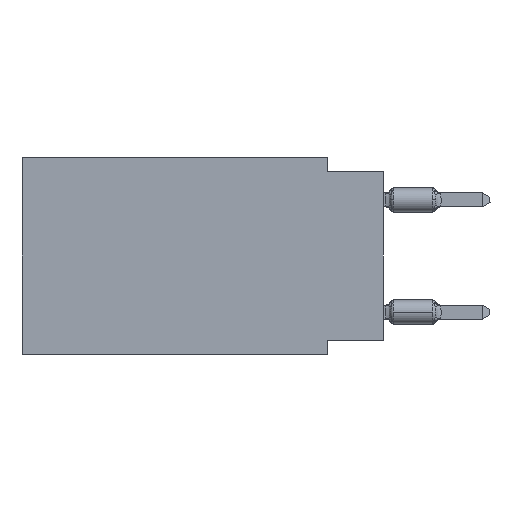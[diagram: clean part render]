
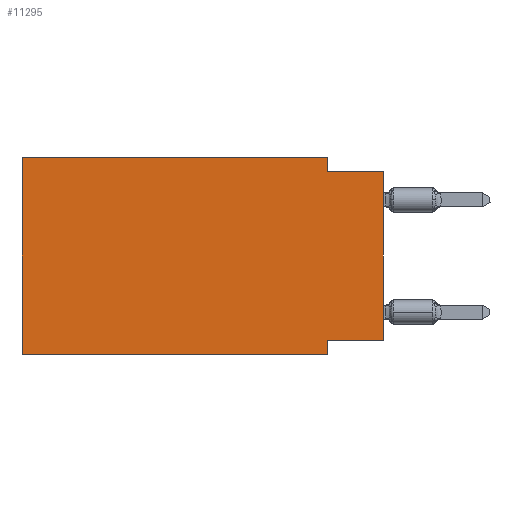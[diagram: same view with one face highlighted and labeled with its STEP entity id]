
A CAD part, left-side view. The second image highlights one B-rep face of the part: STEP entity #11295.
In plain terms, the highlighted planar face has unit normal (-1, 0, 0).
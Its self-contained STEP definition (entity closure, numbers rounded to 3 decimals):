
#116 = LINE ( 'NONE', #10203, #14946 ) ;
#575 = CARTESIAN_POINT ( 'NONE',  ( 0., 16.383, 0. ) ) ;
#640 = CARTESIAN_POINT ( 'NONE',  ( 0., 0., -0.635 ) ) ;
#756 = CARTESIAN_POINT ( 'NONE',  ( 0., 16.383, 0. ) ) ;
#851 = VERTEX_POINT ( 'NONE', #13992 ) ;
#1028 = CARTESIAN_POINT ( 'NONE',  ( 0., 16.383, -8.89 ) ) ;
#1067 = DIRECTION ( 'NONE',  ( 0., 0., -1. ) ) ;
#1612 = ORIENTED_EDGE ( 'NONE', *, *, #9299, .T. ) ;
#1978 = CARTESIAN_POINT ( 'NONE',  ( 0., 0., -8.255 ) ) ;
#2279 = LINE ( 'NONE', #756, #11150 ) ;
#2383 = CARTESIAN_POINT ( 'NONE',  ( 0., 2.54, -8.89 ) ) ;
#2722 = CARTESIAN_POINT ( 'NONE',  ( 0., 16.383, 0. ) ) ;
#2803 = VECTOR ( 'NONE', #16904, 1000. ) ;
#2999 = LINE ( 'NONE', #9617, #2803 ) ;
#3712 = CARTESIAN_POINT ( 'NONE',  ( 0., 16.383, -8.89 ) ) ;
#4449 = VERTEX_POINT ( 'NONE', #640 ) ;
#5041 = CARTESIAN_POINT ( 'NONE',  ( 0., 16.383, 0. ) ) ;
#5807 = VECTOR ( 'NONE', #8614, 1000. ) ;
#5881 = FACE_OUTER_BOUND ( 'NONE', #18463, .T. ) ;
#6036 = ORIENTED_EDGE ( 'NONE', *, *, #7440, .T. ) ;
#7087 = CARTESIAN_POINT ( 'NONE',  ( 0., 2.54, 0. ) ) ;
#7278 = VERTEX_POINT ( 'NONE', #1978 ) ;
#7440 = EDGE_CURVE ( 'NONE', #7278, #4449, #15448, .T. ) ;
#7519 = DIRECTION ( 'NONE',  ( 0., 0., -1. ) ) ;
#7767 = EDGE_CURVE ( 'NONE', #20010, #851, #116, .T. ) ;
#7990 = ORIENTED_EDGE ( 'NONE', *, *, #14927, .F. ) ;
#8484 = VERTEX_POINT ( 'NONE', #3712 ) ;
#8614 = DIRECTION ( 'NONE',  ( 0., 0., 1. ) ) ;
#9299 = EDGE_CURVE ( 'NONE', #8484, #18368, #12979, .T. ) ;
#9408 = EDGE_CURVE ( 'NONE', #851, #4449, #2999, .T. ) ;
#9617 = CARTESIAN_POINT ( 'NONE',  ( 0., 0., -0.635 ) ) ;
#10203 = CARTESIAN_POINT ( 'NONE',  ( 0., 2.54, 0. ) ) ;
#10853 = VERTEX_POINT ( 'NONE', #10909 ) ;
#10909 = CARTESIAN_POINT ( 'NONE',  ( 0., 2.54, -8.255 ) ) ;
#10915 = AXIS2_PLACEMENT_3D ( 'NONE', #575, #13721, #7519 ) ;
#11150 = VECTOR ( 'NONE', #20568, 1000. ) ;
#11295 = ADVANCED_FACE ( 'NONE', ( #5881 ), #20389, .F. ) ;
#12979 = LINE ( 'NONE', #1028, #15638 ) ;
#13254 = VECTOR ( 'NONE', #19060, 1000. ) ;
#13721 = DIRECTION ( 'NONE',  ( 1., 0., 0. ) ) ;
#13770 = ORIENTED_EDGE ( 'NONE', *, *, #19360, .F. ) ;
#13856 = VERTEX_POINT ( 'NONE', #2722 ) ;
#13992 = CARTESIAN_POINT ( 'NONE',  ( 0., 2.54, -0.635 ) ) ;
#14144 = CARTESIAN_POINT ( 'NONE',  ( 0., 0., 0. ) ) ;
#14291 = CARTESIAN_POINT ( 'NONE',  ( 0., 0., -8.255 ) ) ;
#14339 = LINE ( 'NONE', #2383, #19521 ) ;
#14393 = ORIENTED_EDGE ( 'NONE', *, *, #15059, .F. ) ;
#14486 = VECTOR ( 'NONE', #16153, 1000. ) ;
#14724 = LINE ( 'NONE', #14291, #14486 ) ;
#14927 = EDGE_CURVE ( 'NONE', #7278, #10853, #14724, .T. ) ;
#14946 = VECTOR ( 'NONE', #16849, 1000. ) ;
#15059 = EDGE_CURVE ( 'NONE', #8484, #13856, #16784, .T. ) ;
#15374 = CARTESIAN_POINT ( 'NONE',  ( 0., 2.54, -8.89 ) ) ;
#15448 = LINE ( 'NONE', #14144, #13254 ) ;
#15638 = VECTOR ( 'NONE', #21398, 1000. ) ;
#16153 = DIRECTION ( 'NONE',  ( 0., 1., 0. ) ) ;
#16228 = ORIENTED_EDGE ( 'NONE', *, *, #7767, .F. ) ;
#16784 = LINE ( 'NONE', #5041, #5807 ) ;
#16849 = DIRECTION ( 'NONE',  ( 0., 0., -1. ) ) ;
#16904 = DIRECTION ( 'NONE',  ( 0., -1., 0. ) ) ;
#17374 = ORIENTED_EDGE ( 'NONE', *, *, #9408, .F. ) ;
#18368 = VERTEX_POINT ( 'NONE', #15374 ) ;
#18463 = EDGE_LOOP ( 'NONE', ( #6036, #17374, #16228, #18700, #14393, #1612, #13770, #7990 ) ) ;
#18700 = ORIENTED_EDGE ( 'NONE', *, *, #19359, .F. ) ;
#19060 = DIRECTION ( 'NONE',  ( 0., 0., 1. ) ) ;
#19359 = EDGE_CURVE ( 'NONE', #13856, #20010, #2279, .T. ) ;
#19360 = EDGE_CURVE ( 'NONE', #10853, #18368, #14339, .T. ) ;
#19521 = VECTOR ( 'NONE', #1067, 1000. ) ;
#20010 = VERTEX_POINT ( 'NONE', #7087 ) ;
#20389 = PLANE ( 'NONE',  #10915 ) ;
#20568 = DIRECTION ( 'NONE',  ( 0., -1., 0. ) ) ;
#21398 = DIRECTION ( 'NONE',  ( 0., -1., 0. ) ) ;
